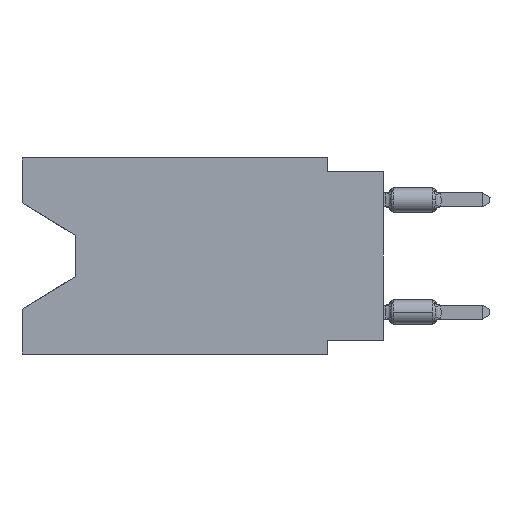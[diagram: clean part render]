
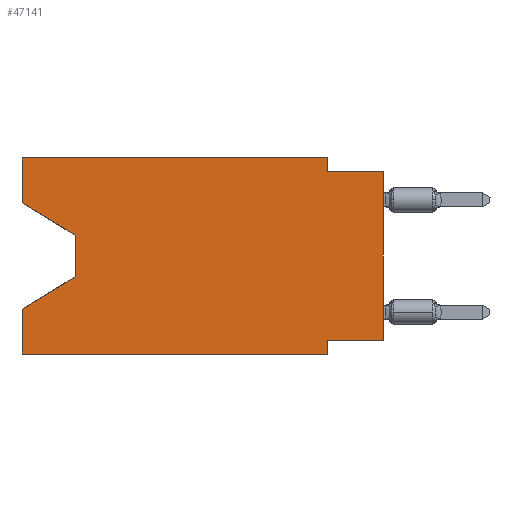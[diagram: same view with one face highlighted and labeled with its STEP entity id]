
A CAD part, left-side view. The second image highlights one B-rep face of the part: STEP entity #47141.
In plain terms, the highlighted planar face has unit normal (-1, 0, 0).
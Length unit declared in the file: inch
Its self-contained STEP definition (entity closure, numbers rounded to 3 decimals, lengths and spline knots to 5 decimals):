
#53 = CARTESIAN_POINT ( 'NONE',  ( 0., 0.645, 0. ) ) ;
#333 = DIRECTION ( 'NONE',  ( 0., 0., 1. ) ) ;
#2366 = LINE ( 'NONE', #19384, #35166 ) ;
#3189 = VERTEX_POINT ( 'NONE', #37976 ) ;
#3641 = EDGE_CURVE ( 'NONE', #4904, #3189, #2366, .T. ) ;
#3701 = FACE_OUTER_BOUND ( 'NONE', #18743, .T. ) ;
#3838 = CARTESIAN_POINT ( 'NONE',  ( 0., 0.1, -0.35 ) ) ;
#3927 = CARTESIAN_POINT ( 'NONE',  ( 0., 0.645, -0.35 ) ) ;
#4136 = VERTEX_POINT ( 'NONE', #8110 ) ;
#4787 = LINE ( 'NONE', #53, #36051 ) ;
#4904 = VERTEX_POINT ( 'NONE', #24966 ) ;
#5346 = DIRECTION ( 'NONE',  ( 0., -0.855, -0.519 ) ) ;
#5645 = VECTOR ( 'NONE', #38944, 39.37008 ) ;
#5817 = VERTEX_POINT ( 'NONE', #3838 ) ;
#6243 = ORIENTED_EDGE ( 'NONE', *, *, #44269, .T. ) ;
#6392 = VECTOR ( 'NONE', #29196, 39.37008 ) ;
#6914 = CARTESIAN_POINT ( 'NONE',  ( 0., 0., -0.325 ) ) ;
#6918 = DIRECTION ( 'NONE',  ( 0., 0., 1. ) ) ;
#8110 = CARTESIAN_POINT ( 'NONE',  ( 0., 0., -0.025 ) ) ;
#8371 = CARTESIAN_POINT ( 'NONE',  ( 0., 0.645, -0.26975 ) ) ;
#8462 = ORIENTED_EDGE ( 'NONE', *, *, #26681, .T. ) ;
#9092 = ORIENTED_EDGE ( 'NONE', *, *, #37117, .F. ) ;
#11792 = CARTESIAN_POINT ( 'NONE',  ( 0., 0.1, 0. ) ) ;
#11801 = PLANE ( 'NONE',  #48183 ) ;
#12337 = DIRECTION ( 'NONE',  ( 1., 0., 0. ) ) ;
#12405 = EDGE_CURVE ( 'NONE', #45673, #31263, #26395, .T. ) ;
#13146 = VERTEX_POINT ( 'NONE', #16354 ) ;
#14377 = VERTEX_POINT ( 'NONE', #31858 ) ;
#14492 = ORIENTED_EDGE ( 'NONE', *, *, #29751, .F. ) ;
#14787 = CARTESIAN_POINT ( 'NONE',  ( 0., 0., -0.025 ) ) ;
#15172 = DIRECTION ( 'NONE',  ( 0., -1., 0. ) ) ;
#15505 = CARTESIAN_POINT ( 'NONE',  ( 0., 0.1, -0.025 ) ) ;
#15789 = LINE ( 'NONE', #31940, #21746 ) ;
#16163 = LINE ( 'NONE', #41553, #30344 ) ;
#16354 = CARTESIAN_POINT ( 'NONE',  ( 0., 0.55, -0.138 ) ) ;
#18743 = EDGE_LOOP ( 'NONE', ( #25561, #6243, #43905, #23380, #36479, #14492, #42277, #8462, #37407, #9092, #19271, #26350 ) ) ;
#19271 = ORIENTED_EDGE ( 'NONE', *, *, #3641, .F. ) ;
#19354 = EDGE_CURVE ( 'NONE', #27422, #5817, #25930, .T. ) ;
#19384 = CARTESIAN_POINT ( 'NONE',  ( 0., 0.645, 0. ) ) ;
#21128 = LINE ( 'NONE', #55057, #44533 ) ;
#21746 = VECTOR ( 'NONE', #44484, 39.37008 ) ;
#21750 = LINE ( 'NONE', #11792, #21789 ) ;
#21789 = VECTOR ( 'NONE', #28797, 39.37008 ) ;
#22617 = LINE ( 'NONE', #22901, #48292 ) ;
#22901 = CARTESIAN_POINT ( 'NONE',  ( 0., 0.645, -0.08025 ) ) ;
#23380 = ORIENTED_EDGE ( 'NONE', *, *, #27828, .F. ) ;
#24264 = VERTEX_POINT ( 'NONE', #49491 ) ;
#24966 = CARTESIAN_POINT ( 'NONE',  ( 0., 0.645, 0. ) ) ;
#25561 = ORIENTED_EDGE ( 'NONE', *, *, #30862, .T. ) ;
#25930 = LINE ( 'NONE', #3927, #49449 ) ;
#26350 = ORIENTED_EDGE ( 'NONE', *, *, #54853, .F. ) ;
#26395 = LINE ( 'NONE', #44199, #5645 ) ;
#26681 = EDGE_CURVE ( 'NONE', #45673, #4136, #16163, .T. ) ;
#26722 = CARTESIAN_POINT ( 'NONE',  ( 0., 0.645, -0.35 ) ) ;
#26764 = LINE ( 'NONE', #14787, #32878 ) ;
#26974 = VERTEX_POINT ( 'NONE', #15505 ) ;
#27422 = VERTEX_POINT ( 'NONE', #26722 ) ;
#27828 = EDGE_CURVE ( 'NONE', #27422, #49434, #21128, .T. ) ;
#28531 = DIRECTION ( 'NONE',  ( 0., 0., -1. ) ) ;
#28797 = DIRECTION ( 'NONE',  ( 0., 0., -1. ) ) ;
#28918 = CARTESIAN_POINT ( 'NONE',  ( 0., 0.1, -0.35 ) ) ;
#29196 = DIRECTION ( 'NONE',  ( 0., 0., -1. ) ) ;
#29731 = DIRECTION ( 'NONE',  ( 0., 0., 1. ) ) ;
#29751 = EDGE_CURVE ( 'NONE', #31263, #5817, #45913, .T. ) ;
#30344 = VECTOR ( 'NONE', #6918, 39.37008 ) ;
#30862 = EDGE_CURVE ( 'NONE', #24264, #13146, #22617, .T. ) ;
#31011 = LINE ( 'NONE', #47175, #54183 ) ;
#31263 = VERTEX_POINT ( 'NONE', #47346 ) ;
#31858 = CARTESIAN_POINT ( 'NONE',  ( 0., 0.55, -0.212 ) ) ;
#31940 = CARTESIAN_POINT ( 'NONE',  ( 0., 0.55, -0.212 ) ) ;
#32878 = VECTOR ( 'NONE', #52918, 39.37008 ) ;
#35166 = VECTOR ( 'NONE', #15172, 39.37008 ) ;
#36051 = VECTOR ( 'NONE', #333, 39.37008 ) ;
#36479 = ORIENTED_EDGE ( 'NONE', *, *, #19354, .T. ) ;
#36516 = EDGE_CURVE ( 'NONE', #14377, #49434, #15789, .T. ) ;
#37117 = EDGE_CURVE ( 'NONE', #3189, #26974, #21750, .T. ) ;
#37407 = ORIENTED_EDGE ( 'NONE', *, *, #44814, .F. ) ;
#37976 = CARTESIAN_POINT ( 'NONE',  ( 0., 0.1, 0. ) ) ;
#38786 = DIRECTION ( 'NONE',  ( 0., -1., 0. ) ) ;
#38944 = DIRECTION ( 'NONE',  ( 0., 1., 0. ) ) ;
#41073 = CARTESIAN_POINT ( 'NONE',  ( 0., 0.645, 0. ) ) ;
#41553 = CARTESIAN_POINT ( 'NONE',  ( 0., 0., 0. ) ) ;
#42277 = ORIENTED_EDGE ( 'NONE', *, *, #12405, .F. ) ;
#43297 = DIRECTION ( 'NONE',  ( 0., 0., -1. ) ) ;
#43905 = ORIENTED_EDGE ( 'NONE', *, *, #36516, .T. ) ;
#44199 = CARTESIAN_POINT ( 'NONE',  ( 0., 0., -0.325 ) ) ;
#44269 = EDGE_CURVE ( 'NONE', #13146, #14377, #31011, .T. ) ;
#44484 = DIRECTION ( 'NONE',  ( 0., 0.855, -0.519 ) ) ;
#44533 = VECTOR ( 'NONE', #29731, 39.37008 ) ;
#44814 = EDGE_CURVE ( 'NONE', #26974, #4136, #26764, .T. ) ;
#45673 = VERTEX_POINT ( 'NONE', #6914 ) ;
#45913 = LINE ( 'NONE', #28918, #6392 ) ;
#47141 = ADVANCED_FACE ( 'NONE', ( #3701 ), #11801, .F. ) ;
#47175 = CARTESIAN_POINT ( 'NONE',  ( 0., 0.55, -0.138 ) ) ;
#47346 = CARTESIAN_POINT ( 'NONE',  ( 0., 0.1, -0.325 ) ) ;
#48183 = AXIS2_PLACEMENT_3D ( 'NONE', #41073, #12337, #28531 ) ;
#48292 = VECTOR ( 'NONE', #5346, 39.37008 ) ;
#49434 = VERTEX_POINT ( 'NONE', #8371 ) ;
#49449 = VECTOR ( 'NONE', #38786, 39.37008 ) ;
#49491 = CARTESIAN_POINT ( 'NONE',  ( 0., 0.645, -0.08025 ) ) ;
#52918 = DIRECTION ( 'NONE',  ( 0., -1., 0. ) ) ;
#54183 = VECTOR ( 'NONE', #43297, 39.37008 ) ;
#54853 = EDGE_CURVE ( 'NONE', #24264, #4904, #4787, .T. ) ;
#55057 = CARTESIAN_POINT ( 'NONE',  ( 0., 0.645, 0. ) ) ;
